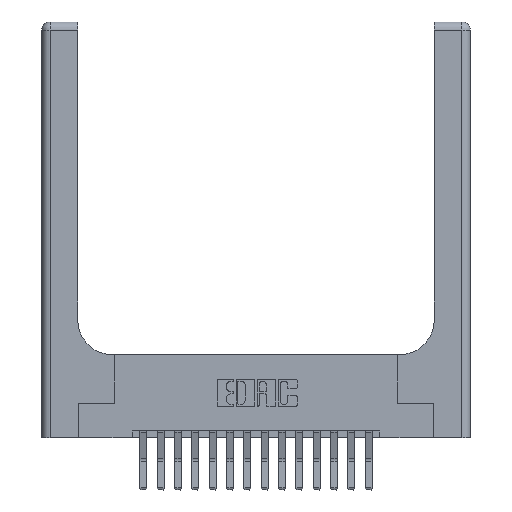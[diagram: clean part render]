
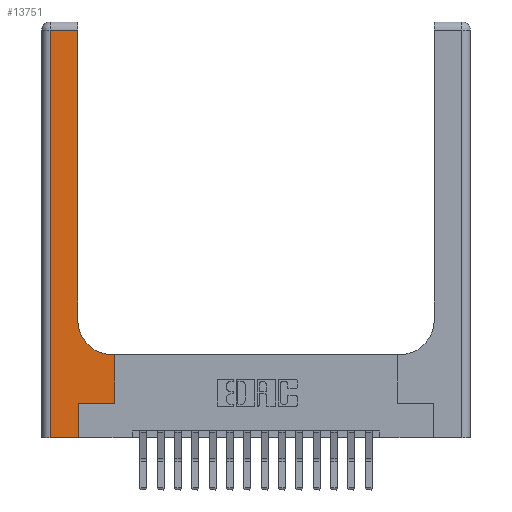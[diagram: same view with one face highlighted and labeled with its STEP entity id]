
A CAD part, top view. The second image highlights one B-rep face of the part: STEP entity #13751.
In plain terms, the highlighted planar face has unit normal (0, 0, 1).
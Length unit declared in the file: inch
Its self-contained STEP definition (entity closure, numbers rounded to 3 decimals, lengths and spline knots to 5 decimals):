
#1 = EDGE_CURVE ( 'NONE', #745, #12116, #3118, .T. ) ;
#26 = ORIENTED_EDGE ( 'NONE', *, *, #13795, .T. ) ;
#72 = CARTESIAN_POINT ( 'NONE',  ( 0., 3., 0.37 ) ) ;
#79 = LINE ( 'NONE', #7340, #12199 ) ;
#200 = VERTEX_POINT ( 'NONE', #9642 ) ;
#402 = CARTESIAN_POINT ( 'NONE',  ( 0.528, 0.25, 0.37 ) ) ;
#745 = VERTEX_POINT ( 'NONE', #9798 ) ;
#773 = EDGE_CURVE ( 'NONE', #17721, #7490, #9480, .T. ) ;
#879 = EDGE_CURVE ( 'NONE', #10849, #1927, #79, .T. ) ;
#1036 = ORIENTED_EDGE ( 'NONE', *, *, #1, .T. ) ;
#1396 = FACE_OUTER_BOUND ( 'NONE', #3287, .T. ) ;
#1452 = ORIENTED_EDGE ( 'NONE', *, *, #16079, .T. ) ;
#1927 = VERTEX_POINT ( 'NONE', #13006 ) ;
#2924 = LINE ( 'NONE', #8794, #14900 ) ;
#2959 = CARTESIAN_POINT ( 'NONE',  ( 0.26, 0.6, 0.37 ) ) ;
#3118 = LINE ( 'NONE', #11816, #3495 ) ;
#3287 = EDGE_LOOP ( 'NONE', ( #26, #1452, #3391, #1036, #9792, #5031, #15358, #16335, #11563 ) ) ;
#3391 = ORIENTED_EDGE ( 'NONE', *, *, #18368, .T. ) ;
#3495 = VECTOR ( 'NONE', #4750, 39.37008 ) ;
#3517 = AXIS2_PLACEMENT_3D ( 'NONE', #72, #11771, #15916 ) ;
#4601 = CARTESIAN_POINT ( 'NONE',  ( 0.26, 3., 0.37 ) ) ;
#4750 = DIRECTION ( 'NONE',  ( 1., 0., 0. ) ) ;
#5031 = ORIENTED_EDGE ( 'NONE', *, *, #11637, .T. ) ;
#5745 = LINE ( 'NONE', #4601, #13762 ) ;
#5809 = LINE ( 'NONE', #2959, #7189 ) ;
#6313 = VECTOR ( 'NONE', #12647, 39.37008 ) ;
#6480 = AXIS2_PLACEMENT_3D ( 'NONE', #11316, #17051, #8490 ) ;
#6893 = CARTESIAN_POINT ( 'NONE',  ( 0.06, 3., 0.37 ) ) ;
#7189 = VECTOR ( 'NONE', #11284, 39.37008 ) ;
#7340 = CARTESIAN_POINT ( 'NONE',  ( 0.528, 0.25, 0.37 ) ) ;
#7405 = LINE ( 'NONE', #13255, #17359 ) ;
#7490 = VERTEX_POINT ( 'NONE', #10126 ) ;
#7910 = EDGE_CURVE ( 'NONE', #12116, #14637, #7405, .T. ) ;
#8490 = DIRECTION ( 'NONE',  ( 1., 0., 0. ) ) ;
#8794 = CARTESIAN_POINT ( 'NONE',  ( 0.265, 0.25, 0.37 ) ) ;
#8796 = CARTESIAN_POINT ( 'NONE',  ( 0.26, 2.94, 0.37 ) ) ;
#9480 = CIRCLE ( 'NONE', #6480, 0.25 ) ;
#9619 = VERTEX_POINT ( 'NONE', #8796 ) ;
#9642 = CARTESIAN_POINT ( 'NONE',  ( 0.06, 2.94, 0.37 ) ) ;
#9792 = ORIENTED_EDGE ( 'NONE', *, *, #7910, .T. ) ;
#9798 = CARTESIAN_POINT ( 'NONE',  ( 0.06, 0., 0.37 ) ) ;
#10126 = CARTESIAN_POINT ( 'NONE',  ( 0.26, 0.85, 0.37 ) ) ;
#10415 = DIRECTION ( 'NONE',  ( 0., 1., 0. ) ) ;
#10849 = VERTEX_POINT ( 'NONE', #402 ) ;
#11284 = DIRECTION ( 'NONE',  ( -1., 0., 0. ) ) ;
#11316 = CARTESIAN_POINT ( 'NONE',  ( 0.51, 0.85, 0.37 ) ) ;
#11563 = ORIENTED_EDGE ( 'NONE', *, *, #773, .T. ) ;
#11637 = EDGE_CURVE ( 'NONE', #14637, #10849, #2924, .T. ) ;
#11721 = DIRECTION ( 'NONE',  ( 1., 0., 0. ) ) ;
#11728 = CARTESIAN_POINT ( 'NONE',  ( 0.265, 0.25, 0.37 ) ) ;
#11771 = DIRECTION ( 'NONE',  ( 0., 0., -1. ) ) ;
#11816 = CARTESIAN_POINT ( 'NONE',  ( 0., 0., 0.37 ) ) ;
#12116 = VERTEX_POINT ( 'NONE', #16212 ) ;
#12119 = DIRECTION ( 'NONE',  ( -1., 0., 0. ) ) ;
#12199 = VECTOR ( 'NONE', #13095, 39.37008 ) ;
#12647 = DIRECTION ( 'NONE',  ( 0., -1., 0. ) ) ;
#13006 = CARTESIAN_POINT ( 'NONE',  ( 0.528, 0.6, 0.37 ) ) ;
#13095 = DIRECTION ( 'NONE',  ( 0., 1., 0. ) ) ;
#13255 = CARTESIAN_POINT ( 'NONE',  ( 0.265, 0., 0.37 ) ) ;
#13281 = PLANE ( 'NONE',  #3517 ) ;
#13751 = ADVANCED_FACE ( 'NONE', ( #1396 ), #13281, .F. ) ;
#13762 = VECTOR ( 'NONE', #16006, 39.37008 ) ;
#13795 = EDGE_CURVE ( 'NONE', #7490, #9619, #5745, .T. ) ;
#14637 = VERTEX_POINT ( 'NONE', #11728 ) ;
#14900 = VECTOR ( 'NONE', #11721, 39.37008 ) ;
#15358 = ORIENTED_EDGE ( 'NONE', *, *, #879, .T. ) ;
#15623 = VECTOR ( 'NONE', #12119, 39.37008 ) ;
#15885 = EDGE_CURVE ( 'NONE', #1927, #17721, #5809, .T. ) ;
#15916 = DIRECTION ( 'NONE',  ( -1., 0., 0. ) ) ;
#16006 = DIRECTION ( 'NONE',  ( 0., 1., 0. ) ) ;
#16079 = EDGE_CURVE ( 'NONE', #9619, #200, #17953, .T. ) ;
#16212 = CARTESIAN_POINT ( 'NONE',  ( 0.265, 0., 0.37 ) ) ;
#16335 = ORIENTED_EDGE ( 'NONE', *, *, #15885, .T. ) ;
#16445 = CARTESIAN_POINT ( 'NONE',  ( 0.51, 0.6, 0.37 ) ) ;
#17051 = DIRECTION ( 'NONE',  ( 0., 0., -1. ) ) ;
#17359 = VECTOR ( 'NONE', #10415, 39.37008 ) ;
#17721 = VERTEX_POINT ( 'NONE', #16445 ) ;
#17953 = LINE ( 'NONE', #18220, #15623 ) ;
#18220 = CARTESIAN_POINT ( 'NONE',  ( 0., 2.94, 0.37 ) ) ;
#18368 = EDGE_CURVE ( 'NONE', #200, #745, #18458, .T. ) ;
#18458 = LINE ( 'NONE', #6893, #6313 ) ;
